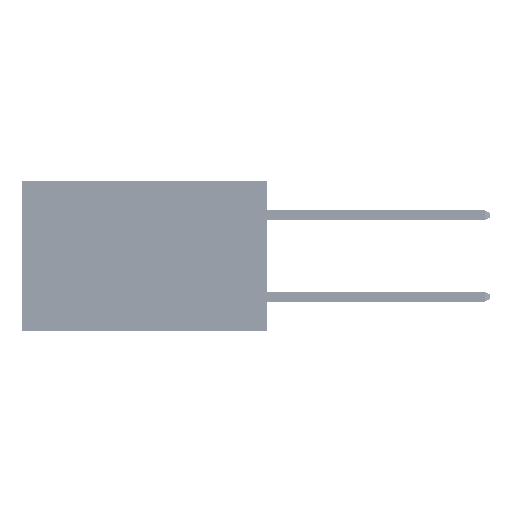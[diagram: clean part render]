
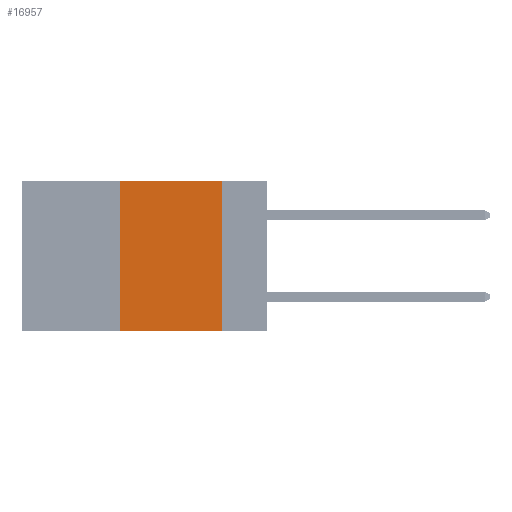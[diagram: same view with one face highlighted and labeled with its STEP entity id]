
A CAD part, left-side view. The second image highlights one B-rep face of the part: STEP entity #16957.
In plain terms, the highlighted planar face has unit normal (-1, 0, 0).
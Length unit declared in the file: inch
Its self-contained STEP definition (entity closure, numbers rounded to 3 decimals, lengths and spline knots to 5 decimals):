
#630 = EDGE_CURVE ( 'NONE', #48953, #14110, #47055, .T. ) ;
#2068 = CARTESIAN_POINT ( 'NONE',  ( 0., 0.11, 0. ) ) ;
#3003 = VECTOR ( 'NONE', #48402, 39.37008 ) ;
#3979 = VECTOR ( 'NONE', #13385, 39.37008 ) ;
#5817 = CARTESIAN_POINT ( 'NONE',  ( 0., 0.36, 0. ) ) ;
#8511 = DIRECTION ( 'NONE',  ( 0., -1., 0. ) ) ;
#9452 = ORIENTED_EDGE ( 'NONE', *, *, #630, .F. ) ;
#12899 = EDGE_CURVE ( 'NONE', #30956, #14110, #34136, .T. ) ;
#13385 = DIRECTION ( 'NONE',  ( 0., 0., 1. ) ) ;
#14110 = VERTEX_POINT ( 'NONE', #45866 ) ;
#15596 = CARTESIAN_POINT ( 'NONE',  ( 0., 0.6, 0. ) ) ;
#15887 = ORIENTED_EDGE ( 'NONE', *, *, #30895, .F. ) ;
#16957 = ADVANCED_FACE ( 'NONE', ( #20472 ), #30911, .F. ) ;
#19320 = LINE ( 'NONE', #35548, #30758 ) ;
#19642 = LINE ( 'NONE', #5817, #3979 ) ;
#20017 = CARTESIAN_POINT ( 'NONE',  ( 0., 0.36, 0. ) ) ;
#20472 = FACE_OUTER_BOUND ( 'NONE', #27991, .T. ) ;
#23460 = VERTEX_POINT ( 'NONE', #20017 ) ;
#24256 = DIRECTION ( 'NONE',  ( 0., -1., 0. ) ) ;
#27386 = CARTESIAN_POINT ( 'NONE',  ( 0., 0.6, -0.37 ) ) ;
#27514 = VECTOR ( 'NONE', #8511, 39.37008 ) ;
#27991 = EDGE_LOOP ( 'NONE', ( #9452, #45659, #15887, #30364 ) ) ;
#30364 = ORIENTED_EDGE ( 'NONE', *, *, #12899, .T. ) ;
#30758 = VECTOR ( 'NONE', #24256, 39.37008 ) ;
#30895 = EDGE_CURVE ( 'NONE', #30956, #23460, #19642, .T. ) ;
#30911 = PLANE ( 'NONE',  #44651 ) ;
#30956 = VERTEX_POINT ( 'NONE', #36952 ) ;
#34136 = LINE ( 'NONE', #27386, #27514 ) ;
#34144 = CARTESIAN_POINT ( 'NONE',  ( 0., 0.11, 0. ) ) ;
#34428 = EDGE_CURVE ( 'NONE', #23460, #48953, #19320, .T. ) ;
#35548 = CARTESIAN_POINT ( 'NONE',  ( 0., 0.6, 0. ) ) ;
#36952 = CARTESIAN_POINT ( 'NONE',  ( 0., 0.36, -0.37 ) ) ;
#42539 = DIRECTION ( 'NONE',  ( 1., 0., 0. ) ) ;
#44651 = AXIS2_PLACEMENT_3D ( 'NONE', #15596, #42539, #46435 ) ;
#45659 = ORIENTED_EDGE ( 'NONE', *, *, #34428, .F. ) ;
#45866 = CARTESIAN_POINT ( 'NONE',  ( 0., 0.11, -0.37 ) ) ;
#46435 = DIRECTION ( 'NONE',  ( 0., 0., -1. ) ) ;
#47055 = LINE ( 'NONE', #2068, #3003 ) ;
#48402 = DIRECTION ( 'NONE',  ( 0., 0., -1. ) ) ;
#48953 = VERTEX_POINT ( 'NONE', #34144 ) ;
